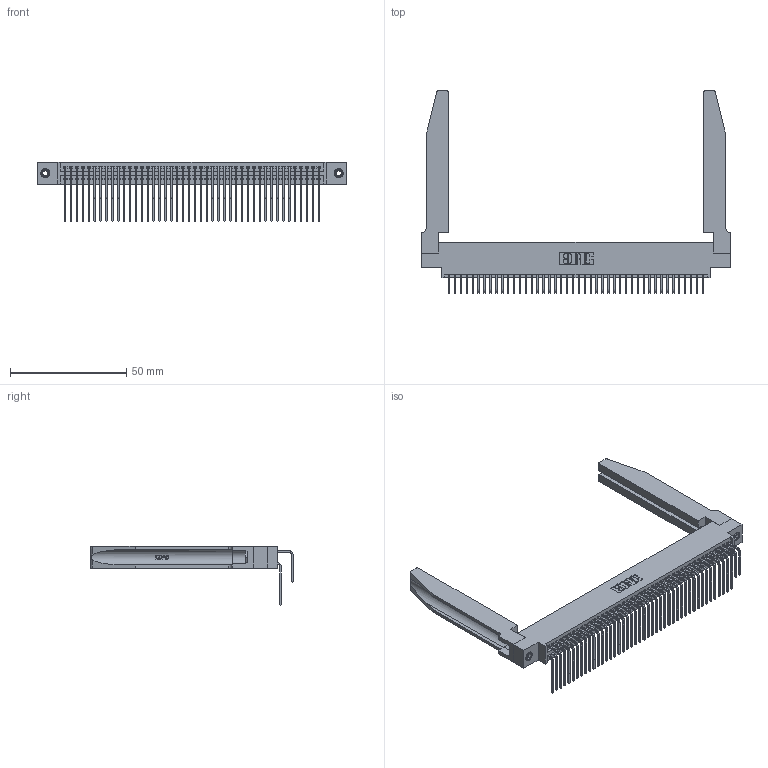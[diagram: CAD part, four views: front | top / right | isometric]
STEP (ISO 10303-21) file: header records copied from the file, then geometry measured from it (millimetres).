
FILE_DESCRIPTION (( 'STEP AP203' ), '1' );
FILE_NAME ('345-088-558-878.STEP', '2019-11-01T13:55:39', ( '' ), ( '' ), 'SwSTEP 2.0', 'SolidWorks 2016', '' );
FILE_SCHEMA (( 'CONFIG_CONTROL_DESIGN' ));
Length unit declared in the file: inch
Products named in the file (6): 345 Part_0.170 Offset - 0.156 Dia-TH; 345-088-558-878; 345-292-001_558 Tail - 2; 345-220-078_345-220-078; 345-292-001_558 559 Tail - 1; 345-250-001_345-250-001-102
Assembly tree (93 placements, depth 2):
  345-088-558-878
    345 Part_0.170 Offset - 0.156 Dia-TH
    345-292-001_558 559 Tail - 1  x44
    345-292-001_558 Tail - 2  x44
    345-250-001_345-250-001-102  x2
    345-220-078_345-220-078  x2
Bounding box: 132.99 x 87.11 x 25.53 mm (x, y, z)
Volume: 21102.5 mm3; surface area: 29114.8 mm2
Topology: 93 solids, 93 shells, 4940 faces, 14601 edges, 9606 vertices
Faces by surface type: plane 3306, cylinder 1582, bspline 36, cone 12, torus 4
Entity records: 40778 total; most frequent: CARTESIAN_POINT 7798, ORIENTED_EDGE 6578, DIRECTION 5839, EDGE_CURVE 3289, VECTOR 2847, LINE 2847, VERTEX_POINT 2184, AXIS2_PLACEMENT_3D 1496
